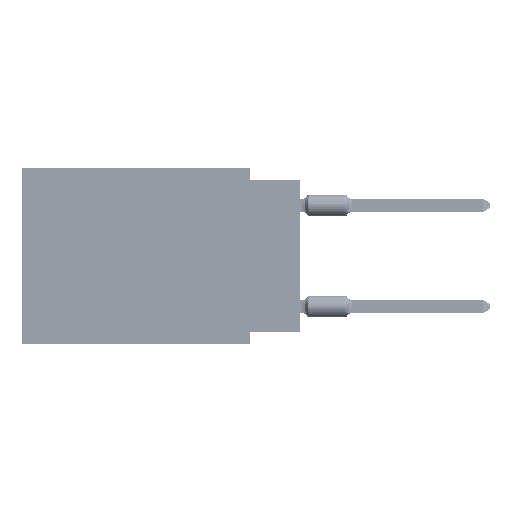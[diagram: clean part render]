
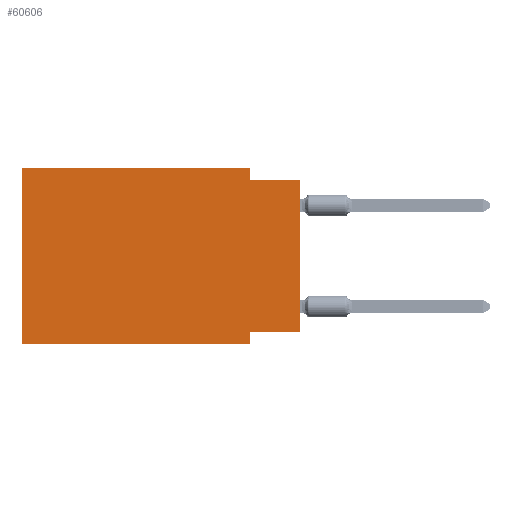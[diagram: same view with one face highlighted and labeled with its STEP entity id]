
A CAD part, left-side view. The second image highlights one B-rep face of the part: STEP entity #60606.
In plain terms, the highlighted planar face has unit normal (-1, 0, 0).
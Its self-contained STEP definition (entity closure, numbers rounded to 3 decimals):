
#1223 = CARTESIAN_POINT ( 'NONE',  ( 0., 2.54, -8.89 ) ) ;
#2931 = DIRECTION ( 'NONE',  ( 0., 0., -1. ) ) ;
#3795 = EDGE_CURVE ( 'NONE', #69957, #33056, #82782, .T. ) ;
#10123 = EDGE_CURVE ( 'NONE', #18246, #51111, #62664, .T. ) ;
#10234 = CARTESIAN_POINT ( 'NONE',  ( 0., 0., -0.635 ) ) ;
#13453 = CARTESIAN_POINT ( 'NONE',  ( 0., 0., 0. ) ) ;
#14344 = VECTOR ( 'NONE', #27482, 1000. ) ;
#14553 = ORIENTED_EDGE ( 'NONE', *, *, #10123, .F. ) ;
#15417 = DIRECTION ( 'NONE',  ( 0., 0., 1. ) ) ;
#16967 = ORIENTED_EDGE ( 'NONE', *, *, #3795, .F. ) ;
#17239 = LINE ( 'NONE', #10234, #72453 ) ;
#17491 = DIRECTION ( 'NONE',  ( 0., 0., -1. ) ) ;
#17976 = VECTOR ( 'NONE', #69171, 1000. ) ;
#18246 = VERTEX_POINT ( 'NONE', #48519 ) ;
#20127 = ORIENTED_EDGE ( 'NONE', *, *, #71473, .F. ) ;
#22042 = CARTESIAN_POINT ( 'NONE',  ( 0., 2.54, -0.635 ) ) ;
#22170 = ORIENTED_EDGE ( 'NONE', *, *, #84934, .F. ) ;
#27482 = DIRECTION ( 'NONE',  ( 0., 0., 1. ) ) ;
#30623 = EDGE_CURVE ( 'NONE', #40565, #37002, #17239, .T. ) ;
#31698 = VERTEX_POINT ( 'NONE', #58397 ) ;
#32680 = DIRECTION ( 'NONE',  ( 0., 0., -1. ) ) ;
#33056 = VERTEX_POINT ( 'NONE', #43773 ) ;
#36189 = CARTESIAN_POINT ( 'NONE',  ( 0., 0., -0.635 ) ) ;
#37002 = VERTEX_POINT ( 'NONE', #36189 ) ;
#38524 = DIRECTION ( 'NONE',  ( 1., 0., 0. ) ) ;
#38753 = LINE ( 'NONE', #83112, #63150 ) ;
#40565 = VERTEX_POINT ( 'NONE', #22042 ) ;
#40671 = CARTESIAN_POINT ( 'NONE',  ( 0., 13.97, 0. ) ) ;
#43773 = CARTESIAN_POINT ( 'NONE',  ( 0., 2.54, -8.89 ) ) ;
#44268 = VECTOR ( 'NONE', #77678, 1000. ) ;
#45321 = CARTESIAN_POINT ( 'NONE',  ( 0., 13.97, -8.89 ) ) ;
#48498 = ORIENTED_EDGE ( 'NONE', *, *, #30623, .F. ) ;
#48519 = CARTESIAN_POINT ( 'NONE',  ( 0., 13.97, -8.89 ) ) ;
#48737 = LINE ( 'NONE', #84699, #44268 ) ;
#48868 = ORIENTED_EDGE ( 'NONE', *, *, #89781, .T. ) ;
#49436 = LINE ( 'NONE', #13453, #14344 ) ;
#51111 = VERTEX_POINT ( 'NONE', #65652 ) ;
#54080 = EDGE_LOOP ( 'NONE', ( #48868, #48498, #22170, #64430, #14553, #75554, #16967, #20127 ) ) ;
#54401 = VECTOR ( 'NONE', #2931, 1000. ) ;
#58397 = CARTESIAN_POINT ( 'NONE',  ( 0., 2.54, 0. ) ) ;
#60606 = ADVANCED_FACE ( 'NONE', ( #67014 ), #81933, .F. ) ;
#62664 = LINE ( 'NONE', #91142, #76156 ) ;
#63150 = VECTOR ( 'NONE', #32680, 1000. ) ;
#63511 = CARTESIAN_POINT ( 'NONE',  ( 0., 0., -8.255 ) ) ;
#64430 = ORIENTED_EDGE ( 'NONE', *, *, #66956, .F. ) ;
#65652 = CARTESIAN_POINT ( 'NONE',  ( 0., 13.97, 0. ) ) ;
#66956 = EDGE_CURVE ( 'NONE', #51111, #31698, #76168, .T. ) ;
#67014 = FACE_OUTER_BOUND ( 'NONE', #54080, .T. ) ;
#67231 = DIRECTION ( 'NONE',  ( 0., -1., 0. ) ) ;
#68395 = CARTESIAN_POINT ( 'NONE',  ( 0., 13.97, 0. ) ) ;
#69171 = DIRECTION ( 'NONE',  ( 0., -1., 0. ) ) ;
#69957 = VERTEX_POINT ( 'NONE', #86604 ) ;
#71473 = EDGE_CURVE ( 'NONE', #80041, #69957, #48737, .T. ) ;
#72453 = VECTOR ( 'NONE', #67231, 1000. ) ;
#72885 = LINE ( 'NONE', #45321, #73375 ) ;
#73375 = VECTOR ( 'NONE', #87341, 1000. ) ;
#75554 = ORIENTED_EDGE ( 'NONE', *, *, #84704, .T. ) ;
#76156 = VECTOR ( 'NONE', #15417, 1000. ) ;
#76168 = LINE ( 'NONE', #40671, #17976 ) ;
#77678 = DIRECTION ( 'NONE',  ( 0., 1., 0. ) ) ;
#80041 = VERTEX_POINT ( 'NONE', #63511 ) ;
#81933 = PLANE ( 'NONE',  #86069 ) ;
#82782 = LINE ( 'NONE', #1223, #54401 ) ;
#83112 = CARTESIAN_POINT ( 'NONE',  ( 0., 2.54, 0. ) ) ;
#84699 = CARTESIAN_POINT ( 'NONE',  ( 0., 0., -8.255 ) ) ;
#84704 = EDGE_CURVE ( 'NONE', #18246, #33056, #72885, .T. ) ;
#84934 = EDGE_CURVE ( 'NONE', #31698, #40565, #38753, .T. ) ;
#86069 = AXIS2_PLACEMENT_3D ( 'NONE', #68395, #38524, #17491 ) ;
#86604 = CARTESIAN_POINT ( 'NONE',  ( 0., 2.54, -8.255 ) ) ;
#87341 = DIRECTION ( 'NONE',  ( 0., -1., 0. ) ) ;
#89781 = EDGE_CURVE ( 'NONE', #80041, #37002, #49436, .T. ) ;
#91142 = CARTESIAN_POINT ( 'NONE',  ( 0., 13.97, 0. ) ) ;
